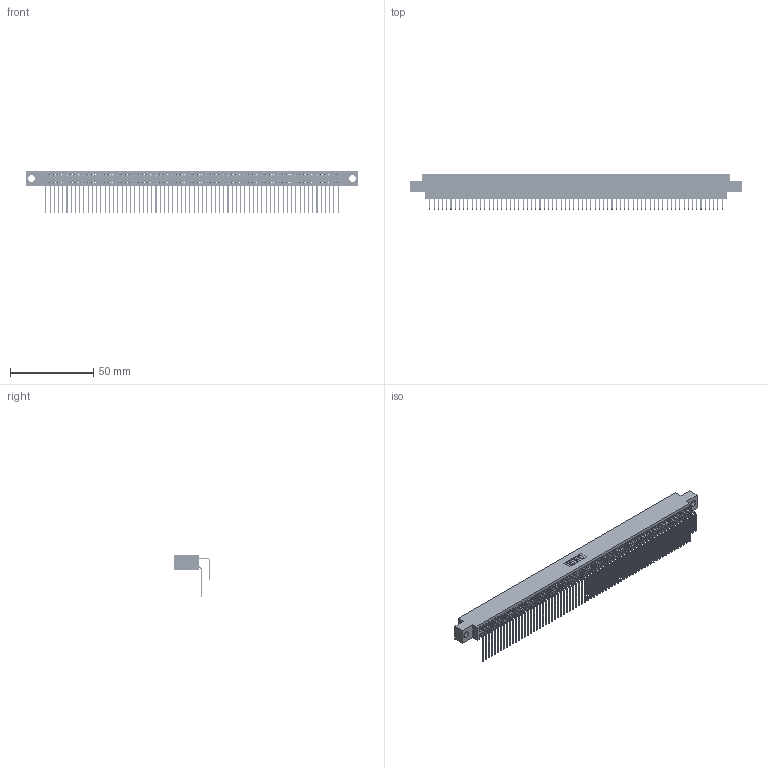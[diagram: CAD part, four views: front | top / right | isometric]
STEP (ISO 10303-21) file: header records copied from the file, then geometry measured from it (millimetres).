
FILE_DESCRIPTION (( 'STEP AP203' ), '1' );
FILE_NAME ('345-140-558-804.STEP', '2021-05-26T01:22:57', ( '' ), ( '' ), 'SwSTEP 2.0', 'SolidWorks 2020', '' );
FILE_SCHEMA (( 'CONFIG_CONTROL_DESIGN' ));
Length unit declared in the file: inch
Products named in the file (4): 345-292-001_558 559 Tail - 1; 345-140-558-804; 345-292-001_558 Tail - 2; 345 Part_0.170 Offset - 0.156 Dia-TI
Assembly tree (141 placements, depth 2):
  345-140-558-804
    345 Part_0.170 Offset - 0.156 Dia-TI
    345-292-001_558 559 Tail - 1  x70
    345-292-001_558 Tail - 2  x70
Bounding box: 199.01 x 21.83 x 25.53 mm (x, y, z)
Volume: 20180.1 mm3; surface area: 34164.7 mm2
Topology: 141 solids, 141 shells, 7424 faces, 22089 edges, 14538 vertices
Faces by surface type: plane 4998, cylinder 2426
Entity records: 53357 total; most frequent: CARTESIAN_POINT 8969, ORIENTED_EDGE 8850, DIRECTION 7845, EDGE_CURVE 4425, LINE 3973, VECTOR 3973, VERTEX_POINT 2946, AXIS2_PLACEMENT_3D 1936
